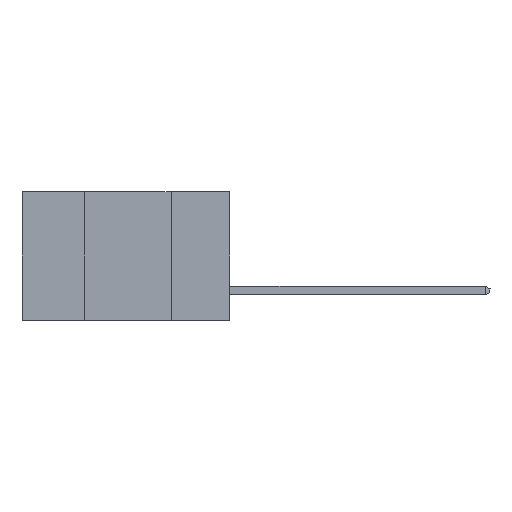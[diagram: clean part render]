
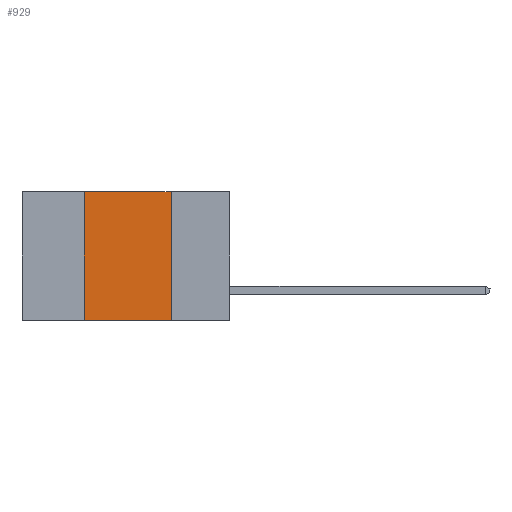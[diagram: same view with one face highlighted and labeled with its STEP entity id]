
A CAD part, left-side view. The second image highlights one B-rep face of the part: STEP entity #929.
In plain terms, the highlighted planar face has unit normal (-1, 0, 0).
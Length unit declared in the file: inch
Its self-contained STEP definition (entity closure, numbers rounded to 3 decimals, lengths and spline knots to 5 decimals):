
#189 = ORIENTED_EDGE ( 'NONE', *, *, #7320, .F. ) ;
#415 = EDGE_CURVE ( 'NONE', #3558, #3318, #7749, .T. ) ;
#702 = CARTESIAN_POINT ( 'NONE',  ( 0., 0.42, -0.37 ) ) ;
#929 = ADVANCED_FACE ( 'NONE', ( #8218 ), #1884, .F. ) ;
#1176 = DIRECTION ( 'NONE',  ( 0., 0., -1. ) ) ;
#1283 = LINE ( 'NONE', #6836, #7448 ) ;
#1724 = VERTEX_POINT ( 'NONE', #2599 ) ;
#1884 = PLANE ( 'NONE',  #4697 ) ;
#2188 = ORIENTED_EDGE ( 'NONE', *, *, #4161, .T. ) ;
#2599 = CARTESIAN_POINT ( 'NONE',  ( 0., 0.42, 0. ) ) ;
#2643 = DIRECTION ( 'NONE',  ( 0., 0., -1. ) ) ;
#2665 = DIRECTION ( 'NONE',  ( 0., -1., 0. ) ) ;
#2706 = CARTESIAN_POINT ( 'NONE',  ( 0., 0.6, 0. ) ) ;
#3318 = VERTEX_POINT ( 'NONE', #7879 ) ;
#3479 = DIRECTION ( 'NONE',  ( 0., -1., 0. ) ) ;
#3558 = VERTEX_POINT ( 'NONE', #6657 ) ;
#3972 = VECTOR ( 'NONE', #5133, 39.37008 ) ;
#4000 = VECTOR ( 'NONE', #2643, 39.37008 ) ;
#4142 = CARTESIAN_POINT ( 'NONE',  ( 0., 0.42, -0.37 ) ) ;
#4161 = EDGE_CURVE ( 'NONE', #5225, #3318, #1283, .T. ) ;
#4378 = VECTOR ( 'NONE', #2665, 39.37008 ) ;
#4697 = AXIS2_PLACEMENT_3D ( 'NONE', #7561, #9031, #1176 ) ;
#4934 = EDGE_CURVE ( 'NONE', #1724, #3558, #5442, .T. ) ;
#5050 = LINE ( 'NONE', #702, #3972 ) ;
#5133 = DIRECTION ( 'NONE',  ( 0., 0., 1. ) ) ;
#5225 = VERTEX_POINT ( 'NONE', #4142 ) ;
#5442 = LINE ( 'NONE', #2706, #4378 ) ;
#6425 = ORIENTED_EDGE ( 'NONE', *, *, #4934, .F. ) ;
#6657 = CARTESIAN_POINT ( 'NONE',  ( 0., 0.17, 0. ) ) ;
#6703 = EDGE_LOOP ( 'NONE', ( #8724, #6425, #189, #2188 ) ) ;
#6836 = CARTESIAN_POINT ( 'NONE',  ( 0., 0.6, -0.37 ) ) ;
#7320 = EDGE_CURVE ( 'NONE', #5225, #1724, #5050, .T. ) ;
#7448 = VECTOR ( 'NONE', #3479, 39.37008 ) ;
#7561 = CARTESIAN_POINT ( 'NONE',  ( 0., 0.6, 0. ) ) ;
#7749 = LINE ( 'NONE', #8374, #4000 ) ;
#7879 = CARTESIAN_POINT ( 'NONE',  ( 0., 0.17, -0.37 ) ) ;
#8218 = FACE_OUTER_BOUND ( 'NONE', #6703, .T. ) ;
#8374 = CARTESIAN_POINT ( 'NONE',  ( 0., 0.17, -0.37 ) ) ;
#8724 = ORIENTED_EDGE ( 'NONE', *, *, #415, .F. ) ;
#9031 = DIRECTION ( 'NONE',  ( 1., 0., 0. ) ) ;
